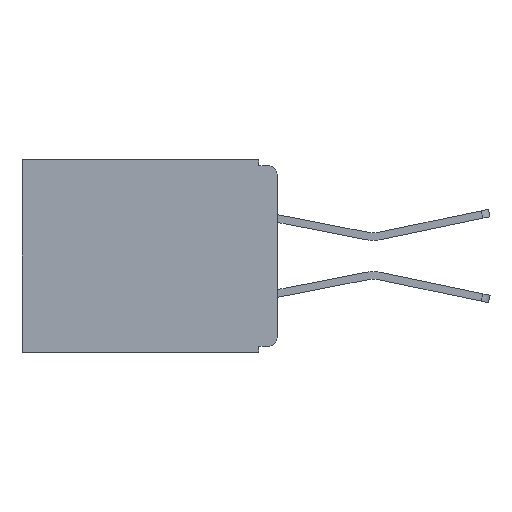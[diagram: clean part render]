
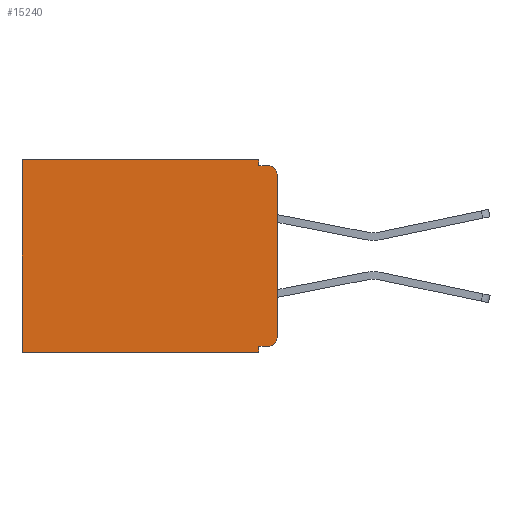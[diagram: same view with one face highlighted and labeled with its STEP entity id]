
A CAD part, left-side view. The second image highlights one B-rep face of the part: STEP entity #15240.
In plain terms, the highlighted planar face has unit normal (-1, 0, 0).
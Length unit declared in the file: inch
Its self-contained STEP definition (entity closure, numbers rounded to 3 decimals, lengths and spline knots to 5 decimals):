
#45 = VECTOR ( 'NONE', #1224, 39.37008 ) ;
#570 = VECTOR ( 'NONE', #4350, 39.37008 ) ;
#1224 = DIRECTION ( 'NONE',  ( 0., 0., -1. ) ) ;
#1683 = VERTEX_POINT ( 'NONE', #4338 ) ;
#1963 = ORIENTED_EDGE ( 'NONE', *, *, #9030, .F. ) ;
#2058 = VECTOR ( 'NONE', #9122, 39.37008 ) ;
#2203 = CARTESIAN_POINT ( 'NONE',  ( 0.3, 0.437, -0.33 ) ) ;
#2372 = EDGE_CURVE ( 'NONE', #11244, #11703, #4188, .T. ) ;
#2399 = AXIS2_PLACEMENT_3D ( 'NONE', #15771, #13222, #13170 ) ;
#2515 = CARTESIAN_POINT ( 'NONE',  ( 0.3, 0.437, -0.33 ) ) ;
#2935 = VERTEX_POINT ( 'NONE', #8428 ) ;
#2976 = DIRECTION ( 'NONE',  ( 0., 0., -1. ) ) ;
#3134 = ORIENTED_EDGE ( 'NONE', *, *, #4506, .T. ) ;
#3201 = DIRECTION ( 'NONE',  ( 1., 0., 0. ) ) ;
#3605 = VECTOR ( 'NONE', #8193, 39.37008 ) ;
#4044 = ORIENTED_EDGE ( 'NONE', *, *, #7234, .T. ) ;
#4188 = LINE ( 'NONE', #13577, #570 ) ;
#4248 = ORIENTED_EDGE ( 'NONE', *, *, #8492, .T. ) ;
#4338 = CARTESIAN_POINT ( 'NONE',  ( 0.3, 0.437, 0. ) ) ;
#4350 = DIRECTION ( 'NONE',  ( 0., 0., -1. ) ) ;
#4444 = DIRECTION ( 'NONE',  ( 0., 1., 0. ) ) ;
#4506 = EDGE_CURVE ( 'NONE', #5760, #11703, #12537, .T. ) ;
#5032 = DIRECTION ( 'NONE',  ( 0., 1., 0. ) ) ;
#5267 = CARTESIAN_POINT ( 'NONE',  ( 0.3, 0.031, -0.32 ) ) ;
#5379 = CIRCLE ( 'NONE', #2399, 0.015 ) ;
#5480 = CARTESIAN_POINT ( 'NONE',  ( 0.3, 0.031, -0.33 ) ) ;
#5760 = VERTEX_POINT ( 'NONE', #11618 ) ;
#6005 = ORIENTED_EDGE ( 'NONE', *, *, #7350, .F. ) ;
#6176 = VECTOR ( 'NONE', #5032, 39.37008 ) ;
#6319 = VECTOR ( 'NONE', #13917, 39.37008 ) ;
#6779 = VECTOR ( 'NONE', #13455, 39.37008 ) ;
#6840 = ORIENTED_EDGE ( 'NONE', *, *, #14363, .F. ) ;
#6893 = DIRECTION ( 'NONE',  ( -1., 0., 0. ) ) ;
#6913 = CARTESIAN_POINT ( 'NONE',  ( 0.3, 0.015, -0.305 ) ) ;
#7028 = LINE ( 'NONE', #11742, #6176 ) ;
#7193 = LINE ( 'NONE', #5480, #6779 ) ;
#7234 = EDGE_CURVE ( 'NONE', #11244, #13314, #5379, .T. ) ;
#7238 = LINE ( 'NONE', #16103, #3605 ) ;
#7273 = VECTOR ( 'NONE', #4444, 39.37008 ) ;
#7350 = EDGE_CURVE ( 'NONE', #12116, #17137, #10855, .T. ) ;
#7693 = AXIS2_PLACEMENT_3D ( 'NONE', #6913, #6893, #2976 ) ;
#8193 = DIRECTION ( 'NONE',  ( 0., -1., 0. ) ) ;
#8242 = EDGE_LOOP ( 'NONE', ( #9104, #4044, #6840, #14130, #13110, #4248, #6005, #13095, #1963, #3134 ) ) ;
#8321 = CARTESIAN_POINT ( 'NONE',  ( 0.3, 0.015, -0.01 ) ) ;
#8428 = CARTESIAN_POINT ( 'NONE',  ( 0.3, 0.031, -0.01 ) ) ;
#8492 = EDGE_CURVE ( 'NONE', #1683, #17137, #14330, .T. ) ;
#9030 = EDGE_CURVE ( 'NONE', #5760, #14896, #7028, .T. ) ;
#9104 = ORIENTED_EDGE ( 'NONE', *, *, #2372, .F. ) ;
#9122 = DIRECTION ( 'NONE',  ( 0., 1., 0. ) ) ;
#10572 = CARTESIAN_POINT ( 'NONE',  ( 0.3, 0.031, 0. ) ) ;
#10855 = LINE ( 'NONE', #14189, #7273 ) ;
#11075 = AXIS2_PLACEMENT_3D ( 'NONE', #11317, #3201, #12656 ) ;
#11244 = VERTEX_POINT ( 'NONE', #12942 ) ;
#11317 = CARTESIAN_POINT ( 'NONE',  ( 0.3, 0., -0.33 ) ) ;
#11353 = EDGE_CURVE ( 'NONE', #17268, #1683, #16271, .T. ) ;
#11618 = CARTESIAN_POINT ( 'NONE',  ( 0.3, 0.015, -0.32 ) ) ;
#11703 = VERTEX_POINT ( 'NONE', #12580 ) ;
#11742 = CARTESIAN_POINT ( 'NONE',  ( 0.3, 0., -0.32 ) ) ;
#12116 = VERTEX_POINT ( 'NONE', #13492 ) ;
#12537 = CIRCLE ( 'NONE', #7693, 0.015 ) ;
#12580 = CARTESIAN_POINT ( 'NONE',  ( 0.3, 0., -0.305 ) ) ;
#12619 = CARTESIAN_POINT ( 'NONE',  ( 0.3, 0.031, 0. ) ) ;
#12656 = DIRECTION ( 'NONE',  ( 0., 0., -1. ) ) ;
#12942 = CARTESIAN_POINT ( 'NONE',  ( 0.3, 0., -0.025 ) ) ;
#13095 = ORIENTED_EDGE ( 'NONE', *, *, #15664, .F. ) ;
#13110 = ORIENTED_EDGE ( 'NONE', *, *, #11353, .T. ) ;
#13170 = DIRECTION ( 'NONE',  ( 0., 0., -1. ) ) ;
#13222 = DIRECTION ( 'NONE',  ( -1., 0., 0. ) ) ;
#13314 = VERTEX_POINT ( 'NONE', #8321 ) ;
#13455 = DIRECTION ( 'NONE',  ( 0., 0., -1. ) ) ;
#13492 = CARTESIAN_POINT ( 'NONE',  ( 0.3, 0.031, -0.33 ) ) ;
#13577 = CARTESIAN_POINT ( 'NONE',  ( 0.3, 0., -0.33 ) ) ;
#13823 = LINE ( 'NONE', #12619, #6319 ) ;
#13917 = DIRECTION ( 'NONE',  ( 0., 0., -1. ) ) ;
#14130 = ORIENTED_EDGE ( 'NONE', *, *, #16535, .F. ) ;
#14189 = CARTESIAN_POINT ( 'NONE',  ( 0.3, 0., -0.33 ) ) ;
#14330 = LINE ( 'NONE', #2515, #45 ) ;
#14363 = EDGE_CURVE ( 'NONE', #2935, #13314, #7238, .T. ) ;
#14452 = CARTESIAN_POINT ( 'NONE',  ( 0.3, 0., 0. ) ) ;
#14896 = VERTEX_POINT ( 'NONE', #5267 ) ;
#15240 = ADVANCED_FACE ( 'NONE', ( #16928 ), #16518, .F. ) ;
#15664 = EDGE_CURVE ( 'NONE', #14896, #12116, #7193, .T. ) ;
#15771 = CARTESIAN_POINT ( 'NONE',  ( 0.3, 0.015, -0.025 ) ) ;
#16103 = CARTESIAN_POINT ( 'NONE',  ( 0.3, 0., -0.01 ) ) ;
#16271 = LINE ( 'NONE', #14452, #2058 ) ;
#16518 = PLANE ( 'NONE',  #11075 ) ;
#16535 = EDGE_CURVE ( 'NONE', #17268, #2935, #13823, .T. ) ;
#16928 = FACE_OUTER_BOUND ( 'NONE', #8242, .T. ) ;
#17137 = VERTEX_POINT ( 'NONE', #2203 ) ;
#17268 = VERTEX_POINT ( 'NONE', #10572 ) ;
